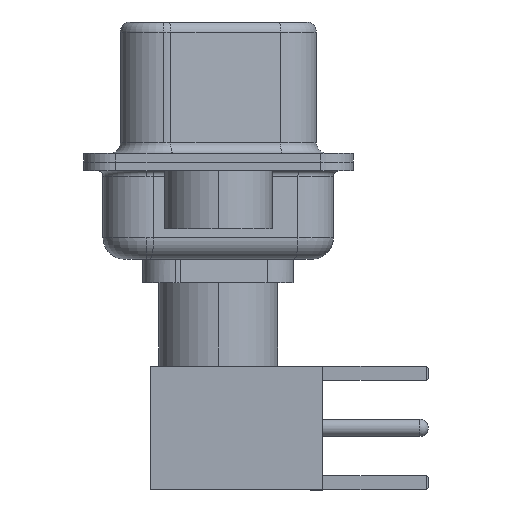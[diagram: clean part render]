
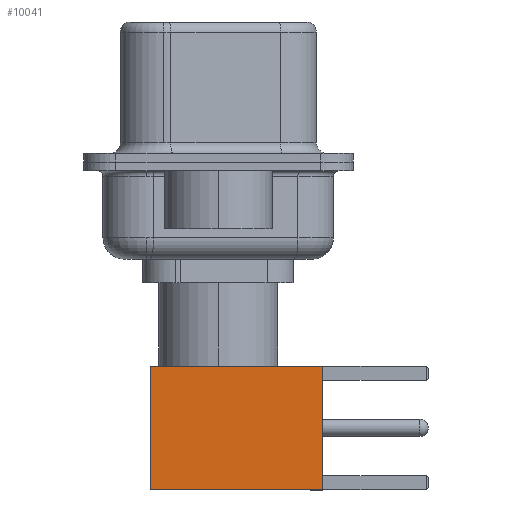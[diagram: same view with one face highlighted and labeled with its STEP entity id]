
A CAD part, left-side view. The second image highlights one B-rep face of the part: STEP entity #10041.
In plain terms, the highlighted face is planar.
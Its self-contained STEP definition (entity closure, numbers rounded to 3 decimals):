
#2032 = ORIENTED_EDGE ( 'NONE', *, *, #8502, .F. ) ;
#2143 = LINE ( 'NONE', #7926, #13820 ) ;
#3866 = PLANE ( 'NONE',  #12721 ) ;
#3955 = VECTOR ( 'NONE', #8809, 1000. ) ;
#4177 = VERTEX_POINT ( 'NONE', #16428 ) ;
#5180 = DIRECTION ( 'NONE',  ( 0., 0., 1. ) ) ;
#5461 = CARTESIAN_POINT ( 'NONE',  ( 2.875, 2.875, 0. ) ) ;
#5678 = VERTEX_POINT ( 'NONE', #18358 ) ;
#6024 = LINE ( 'NONE', #10609, #3955 ) ;
#6346 = DIRECTION ( 'NONE',  ( -1., 0., 0. ) ) ;
#6856 = FACE_OUTER_BOUND ( 'NONE', #10102, .T. ) ;
#6868 = ORIENTED_EDGE ( 'NONE', *, *, #15408, .F. ) ;
#7217 = VECTOR ( 'NONE', #19162, 1000. ) ;
#7926 = CARTESIAN_POINT ( 'NONE',  ( 0., 2.875, 0. ) ) ;
#8261 = VECTOR ( 'NONE', #13651, 1000. ) ;
#8429 = LINE ( 'NONE', #5461, #7217 ) ;
#8502 = EDGE_CURVE ( 'NONE', #13283, #13221, #10772, .T. ) ;
#8809 = DIRECTION ( 'NONE',  ( -1., 0., 0. ) ) ;
#10041 = ADVANCED_FACE ( 'NONE', ( #6856 ), #3866, .T. ) ;
#10102 = EDGE_LOOP ( 'NONE', ( #15053, #19637, #2032, #6868 ) ) ;
#10609 = CARTESIAN_POINT ( 'NONE',  ( 0., 2.875, 8. ) ) ;
#10772 = LINE ( 'NONE', #13946, #8261 ) ;
#12681 = CARTESIAN_POINT ( 'NONE',  ( -2.875, 2.875, 8. ) ) ;
#12721 = AXIS2_PLACEMENT_3D ( 'NONE', #14603, #12833, #5180 ) ;
#12833 = DIRECTION ( 'NONE',  ( 0., 1., 0. ) ) ;
#13221 = VERTEX_POINT ( 'NONE', #15661 ) ;
#13283 = VERTEX_POINT ( 'NONE', #12681 ) ;
#13651 = DIRECTION ( 'NONE',  ( 0., 0., -1. ) ) ;
#13820 = VECTOR ( 'NONE', #6346, 1000. ) ;
#13946 = CARTESIAN_POINT ( 'NONE',  ( -2.875, 2.875, 0. ) ) ;
#14603 = CARTESIAN_POINT ( 'NONE',  ( 2.875, 2.875, 0. ) ) ;
#15053 = ORIENTED_EDGE ( 'NONE', *, *, #19329, .T. ) ;
#15166 = EDGE_CURVE ( 'NONE', #4177, #13221, #2143, .T. ) ;
#15408 = EDGE_CURVE ( 'NONE', #5678, #13283, #6024, .T. ) ;
#15661 = CARTESIAN_POINT ( 'NONE',  ( -2.875, 2.875, 0. ) ) ;
#16428 = CARTESIAN_POINT ( 'NONE',  ( 2.875, 2.875, 0. ) ) ;
#18358 = CARTESIAN_POINT ( 'NONE',  ( 2.875, 2.875, 8. ) ) ;
#19162 = DIRECTION ( 'NONE',  ( 0., 0., -1. ) ) ;
#19329 = EDGE_CURVE ( 'NONE', #5678, #4177, #8429, .T. ) ;
#19637 = ORIENTED_EDGE ( 'NONE', *, *, #15166, .T. ) ;
